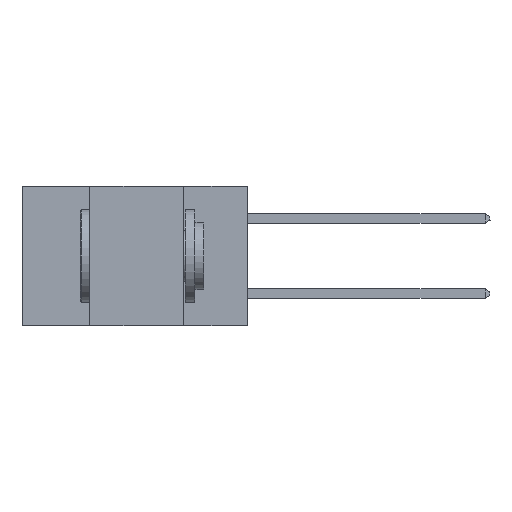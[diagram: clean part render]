
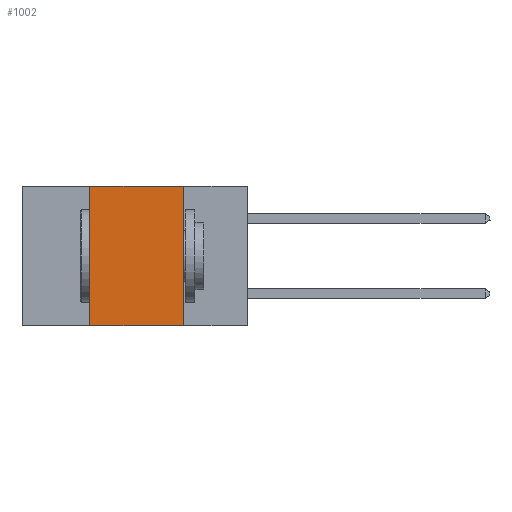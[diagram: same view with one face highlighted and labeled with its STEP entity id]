
A CAD part, left-side view. The second image highlights one B-rep face of the part: STEP entity #1002.
In plain terms, the highlighted planar face has unit normal (-1, 0, 0).
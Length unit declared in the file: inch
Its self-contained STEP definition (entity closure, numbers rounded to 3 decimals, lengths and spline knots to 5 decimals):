
#731 = ORIENTED_EDGE ( 'NONE', *, *, #1757, .F. ) ;
#985 = EDGE_CURVE ( 'NONE', #4201, #3466, #6412, .T. ) ;
#1002 = ADVANCED_FACE ( 'NONE', ( #10031 ), #15489, .F. ) ;
#1757 = EDGE_CURVE ( 'NONE', #5962, #4201, #22812, .T. ) ;
#2449 = ORIENTED_EDGE ( 'NONE', *, *, #12637, .T. ) ;
#3466 = VERTEX_POINT ( 'NONE', #5328 ) ;
#3708 = ORIENTED_EDGE ( 'NONE', *, *, #23051, .F. ) ;
#4201 = VERTEX_POINT ( 'NONE', #6452 ) ;
#5158 = DIRECTION ( 'NONE',  ( 0., -1., 0. ) ) ;
#5328 = CARTESIAN_POINT ( 'NONE',  ( 0., 0.17, -0.37 ) ) ;
#5505 = VECTOR ( 'NONE', #15012, 39.37008 ) ;
#5936 = CARTESIAN_POINT ( 'NONE',  ( 0., 0.6, 0. ) ) ;
#5962 = VERTEX_POINT ( 'NONE', #12704 ) ;
#6412 = LINE ( 'NONE', #21194, #19516 ) ;
#6452 = CARTESIAN_POINT ( 'NONE',  ( 0., 0.17, 0. ) ) ;
#7266 = LINE ( 'NONE', #17964, #11461 ) ;
#9598 = CARTESIAN_POINT ( 'NONE',  ( 0., 0.6, -0.37 ) ) ;
#10031 = FACE_OUTER_BOUND ( 'NONE', #19570, .T. ) ;
#11461 = VECTOR ( 'NONE', #19752, 39.37008 ) ;
#11840 = DIRECTION ( 'NONE',  ( 1., 0., 0. ) ) ;
#12351 = AXIS2_PLACEMENT_3D ( 'NONE', #17139, #11840, #12496 ) ;
#12496 = DIRECTION ( 'NONE',  ( 0., 0., -1. ) ) ;
#12637 = EDGE_CURVE ( 'NONE', #19604, #3466, #19737, .T. ) ;
#12704 = CARTESIAN_POINT ( 'NONE',  ( 0., 0.42, 0. ) ) ;
#15012 = DIRECTION ( 'NONE',  ( 0., -1., 0. ) ) ;
#15489 = PLANE ( 'NONE',  #12351 ) ;
#17139 = CARTESIAN_POINT ( 'NONE',  ( 0., 0.6, 0. ) ) ;
#17964 = CARTESIAN_POINT ( 'NONE',  ( 0., 0.42, -0.37 ) ) ;
#18075 = VECTOR ( 'NONE', #5158, 39.37008 ) ;
#19516 = VECTOR ( 'NONE', #22404, 39.37008 ) ;
#19570 = EDGE_LOOP ( 'NONE', ( #22656, #731, #3708, #2449 ) ) ;
#19604 = VERTEX_POINT ( 'NONE', #21628 ) ;
#19737 = LINE ( 'NONE', #9598, #5505 ) ;
#19752 = DIRECTION ( 'NONE',  ( 0., 0., 1. ) ) ;
#21194 = CARTESIAN_POINT ( 'NONE',  ( 0., 0.17, -0.37 ) ) ;
#21628 = CARTESIAN_POINT ( 'NONE',  ( 0., 0.42, -0.37 ) ) ;
#22404 = DIRECTION ( 'NONE',  ( 0., 0., -1. ) ) ;
#22656 = ORIENTED_EDGE ( 'NONE', *, *, #985, .F. ) ;
#22812 = LINE ( 'NONE', #5936, #18075 ) ;
#23051 = EDGE_CURVE ( 'NONE', #19604, #5962, #7266, .T. ) ;
